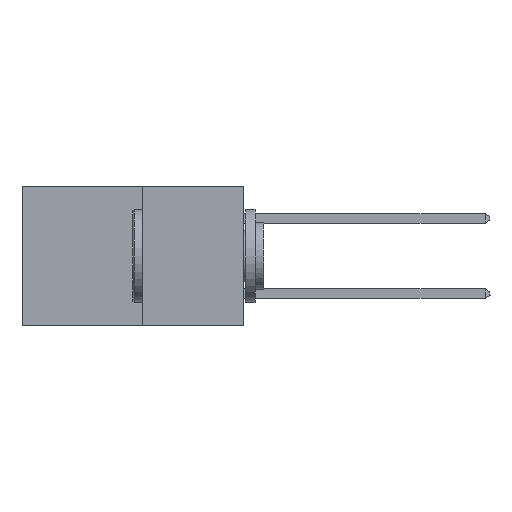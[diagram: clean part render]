
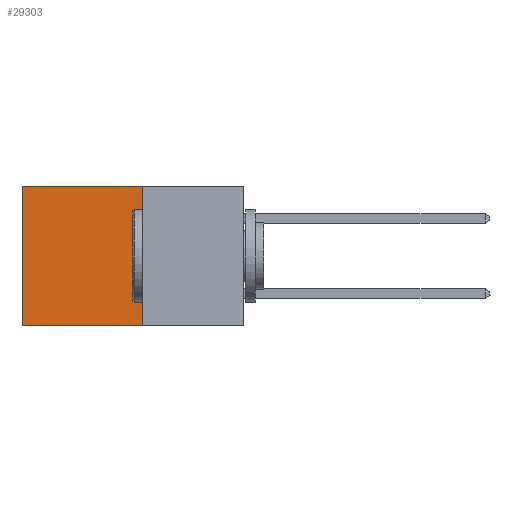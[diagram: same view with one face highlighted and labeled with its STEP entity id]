
A CAD part, left-side view. The second image highlights one B-rep face of the part: STEP entity #29303.
In plain terms, the highlighted planar face has unit normal (-1, 0, 0).
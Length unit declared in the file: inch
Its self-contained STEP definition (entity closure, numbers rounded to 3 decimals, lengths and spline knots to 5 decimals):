
#284 = EDGE_CURVE ( 'NONE', #30874, #10395, #18688, .T. ) ;
#2940 = DIRECTION ( 'NONE',  ( 0., 0., -1. ) ) ;
#3005 = DIRECTION ( 'NONE',  ( 0., 1., 0. ) ) ;
#3610 = ORIENTED_EDGE ( 'NONE', *, *, #29400, .F. ) ;
#4386 = EDGE_CURVE ( 'NONE', #19607, #10395, #19071, .T. ) ;
#4608 = EDGE_LOOP ( 'NONE', ( #6829, #16181, #3610, #19316 ) ) ;
#4613 = FACE_OUTER_BOUND ( 'NONE', #4608, .T. ) ;
#5094 = DIRECTION ( 'NONE',  ( 0., 0., -1. ) ) ;
#5267 = VECTOR ( 'NONE', #20175, 39.37008 ) ;
#6829 = ORIENTED_EDGE ( 'NONE', *, *, #284, .T. ) ;
#7276 = LINE ( 'NONE', #7840, #18790 ) ;
#7618 = EDGE_CURVE ( 'NONE', #11298, #30874, #26700, .T. ) ;
#7840 = CARTESIAN_POINT ( 'NONE',  ( 0.277, 0.27, -0.37 ) ) ;
#9900 = PLANE ( 'NONE',  #17520 ) ;
#10011 = CARTESIAN_POINT ( 'NONE',  ( 0.277, 0.27, 0. ) ) ;
#10395 = VERTEX_POINT ( 'NONE', #12564 ) ;
#11298 = VERTEX_POINT ( 'NONE', #10011 ) ;
#11908 = CARTESIAN_POINT ( 'NONE',  ( 0.277, 0.59, -0.37 ) ) ;
#12137 = VECTOR ( 'NONE', #15700, 39.37008 ) ;
#12564 = CARTESIAN_POINT ( 'NONE',  ( 0.277, 0.59, -0.37 ) ) ;
#12681 = CARTESIAN_POINT ( 'NONE',  ( 0.277, 0.27, 0. ) ) ;
#14807 = CARTESIAN_POINT ( 'NONE',  ( 0.277, 0.27, -0.37 ) ) ;
#15700 = DIRECTION ( 'NONE',  ( 0., 0., -1. ) ) ;
#16181 = ORIENTED_EDGE ( 'NONE', *, *, #4386, .F. ) ;
#16938 = CARTESIAN_POINT ( 'NONE',  ( 0.277, 0.27, -0.37 ) ) ;
#17520 = AXIS2_PLACEMENT_3D ( 'NONE', #14807, #19762, #5094 ) ;
#17693 = CARTESIAN_POINT ( 'NONE',  ( 0.277, 0.27, -0.37 ) ) ;
#18279 = CARTESIAN_POINT ( 'NONE',  ( 0.277, 0.59, 0. ) ) ;
#18688 = LINE ( 'NONE', #11908, #12137 ) ;
#18790 = VECTOR ( 'NONE', #2940, 39.37008 ) ;
#19071 = LINE ( 'NONE', #17693, #5267 ) ;
#19316 = ORIENTED_EDGE ( 'NONE', *, *, #7618, .T. ) ;
#19607 = VERTEX_POINT ( 'NONE', #16938 ) ;
#19762 = DIRECTION ( 'NONE',  ( 1., 0., 0. ) ) ;
#20175 = DIRECTION ( 'NONE',  ( 0., 1., 0. ) ) ;
#25923 = VECTOR ( 'NONE', #3005, 39.37008 ) ;
#26700 = LINE ( 'NONE', #12681, #25923 ) ;
#29303 = ADVANCED_FACE ( 'NONE', ( #4613 ), #9900, .F. ) ;
#29400 = EDGE_CURVE ( 'NONE', #11298, #19607, #7276, .T. ) ;
#30874 = VERTEX_POINT ( 'NONE', #18279 ) ;
